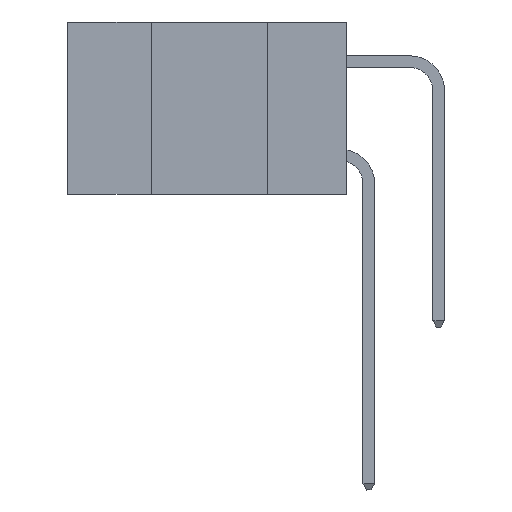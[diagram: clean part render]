
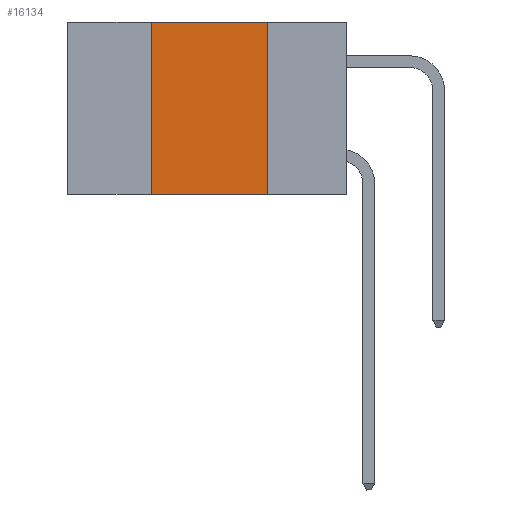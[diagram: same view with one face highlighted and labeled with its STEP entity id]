
A CAD part, left-side view. The second image highlights one B-rep face of the part: STEP entity #16134.
In plain terms, the highlighted planar face has unit normal (-1, 0, 0).
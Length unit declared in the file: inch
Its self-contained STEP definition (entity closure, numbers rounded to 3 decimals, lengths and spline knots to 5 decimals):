
#422 = DIRECTION ( 'NONE',  ( 1., 0., 0. ) ) ;
#1067 = LINE ( 'NONE', #3218, #13006 ) ;
#1791 = DIRECTION ( 'NONE',  ( 0., 0., -1. ) ) ;
#1880 = EDGE_CURVE ( 'NONE', #4885, #11403, #7551, .T. ) ;
#2114 = CARTESIAN_POINT ( 'NONE',  ( 0., 0.42, 0. ) ) ;
#2144 = LINE ( 'NONE', #14495, #9551 ) ;
#2216 = DIRECTION ( 'NONE',  ( 0., 0., 1. ) ) ;
#2240 = ORIENTED_EDGE ( 'NONE', *, *, #10486, .F. ) ;
#2497 = ORIENTED_EDGE ( 'NONE', *, *, #1880, .F. ) ;
#2831 = LINE ( 'NONE', #11887, #3237 ) ;
#3005 = DIRECTION ( 'NONE',  ( 0., -1., 0. ) ) ;
#3218 = CARTESIAN_POINT ( 'NONE',  ( 0., 0.17, 0. ) ) ;
#3237 = VECTOR ( 'NONE', #3005, 39.37008 ) ;
#4885 = VERTEX_POINT ( 'NONE', #15770 ) ;
#6460 = CARTESIAN_POINT ( 'NONE',  ( 0., 0.42, 0. ) ) ;
#7551 = LINE ( 'NONE', #2114, #8779 ) ;
#8256 = EDGE_CURVE ( 'NONE', #11403, #14052, #2144, .T. ) ;
#8779 = VECTOR ( 'NONE', #2216, 39.37008 ) ;
#9551 = VECTOR ( 'NONE', #9895, 39.37008 ) ;
#9895 = DIRECTION ( 'NONE',  ( 0., -1., 0. ) ) ;
#10332 = AXIS2_PLACEMENT_3D ( 'NONE', #15600, #422, #11985 ) ;
#10486 = EDGE_CURVE ( 'NONE', #14052, #16039, #1067, .T. ) ;
#11403 = VERTEX_POINT ( 'NONE', #6460 ) ;
#11654 = CARTESIAN_POINT ( 'NONE',  ( 0., 0.17, 0. ) ) ;
#11702 = EDGE_CURVE ( 'NONE', #4885, #16039, #2831, .T. ) ;
#11887 = CARTESIAN_POINT ( 'NONE',  ( 0., 0.6, -0.37 ) ) ;
#11985 = DIRECTION ( 'NONE',  ( 0., 0., -1. ) ) ;
#12044 = PLANE ( 'NONE',  #10332 ) ;
#12315 = CARTESIAN_POINT ( 'NONE',  ( 0., 0.17, -0.37 ) ) ;
#13006 = VECTOR ( 'NONE', #1791, 39.37008 ) ;
#13074 = ORIENTED_EDGE ( 'NONE', *, *, #11702, .T. ) ;
#13729 = ORIENTED_EDGE ( 'NONE', *, *, #8256, .F. ) ;
#14052 = VERTEX_POINT ( 'NONE', #11654 ) ;
#14495 = CARTESIAN_POINT ( 'NONE',  ( 0., 0.6, 0. ) ) ;
#14678 = EDGE_LOOP ( 'NONE', ( #2240, #13729, #2497, #13074 ) ) ;
#15193 = FACE_OUTER_BOUND ( 'NONE', #14678, .T. ) ;
#15600 = CARTESIAN_POINT ( 'NONE',  ( 0., 0.6, 0. ) ) ;
#15770 = CARTESIAN_POINT ( 'NONE',  ( 0., 0.42, -0.37 ) ) ;
#16039 = VERTEX_POINT ( 'NONE', #12315 ) ;
#16134 = ADVANCED_FACE ( 'NONE', ( #15193 ), #12044, .F. ) ;
